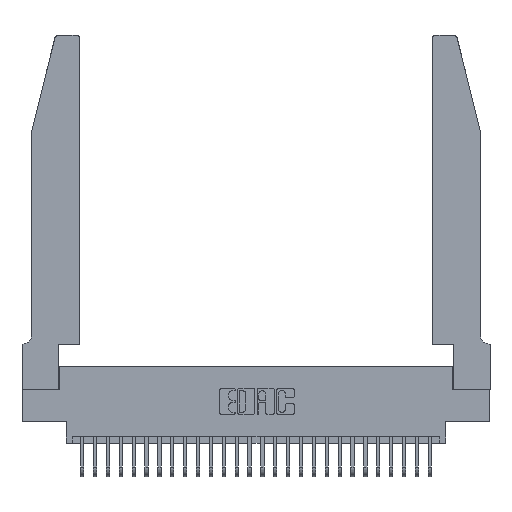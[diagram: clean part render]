
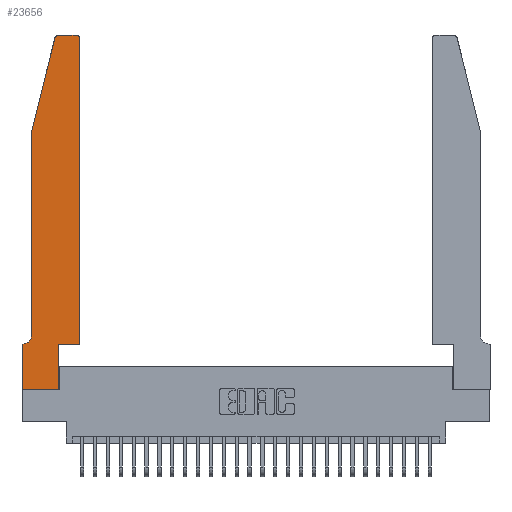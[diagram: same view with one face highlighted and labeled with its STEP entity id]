
A CAD part, top view. The second image highlights one B-rep face of the part: STEP entity #23656.
In plain terms, the highlighted planar face has unit normal (0, 0, 1).
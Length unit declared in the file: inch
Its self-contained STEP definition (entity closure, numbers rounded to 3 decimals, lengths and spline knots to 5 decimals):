
#1052 = DIRECTION ( 'NONE',  ( -1., 0., 0. ) ) ;
#1297 = LINE ( 'NONE', #5480, #9354 ) ;
#1341 = CARTESIAN_POINT ( 'NONE',  ( 0.4505, 0.35, 0.37 ) ) ;
#1685 = EDGE_CURVE ( 'NONE', #15370, #19564, #8620, .T. ) ;
#2724 = CARTESIAN_POINT ( 'NONE',  ( 0.4505, 0.35, 0.37 ) ) ;
#2980 = ORIENTED_EDGE ( 'NONE', *, *, #28537, .T. ) ;
#3102 = CARTESIAN_POINT ( 'NONE',  ( 0.4205, 2.72, 0.37 ) ) ;
#3246 = DIRECTION ( 'NONE',  ( 0., -1., 0. ) ) ;
#3473 = VERTEX_POINT ( 'NONE', #1341 ) ;
#3704 = DIRECTION ( 'NONE',  ( 0., 0., -1. ) ) ;
#3849 = CARTESIAN_POINT ( 'NONE',  ( 0.0755, 2., 0.37 ) ) ;
#4009 = EDGE_CURVE ( 'NONE', #21782, #7893, #15724, .T. ) ;
#4405 = EDGE_CURVE ( 'NONE', #24152, #15370, #26094, .T. ) ;
#5164 = CIRCLE ( 'NONE', #14591, 0.03 ) ;
#5480 = CARTESIAN_POINT ( 'NONE',  ( 0., 0., 0.37 ) ) ;
#5598 = ORIENTED_EDGE ( 'NONE', *, *, #10069, .T. ) ;
#6657 = DIRECTION ( 'NONE',  ( 0., 0., 1. ) ) ;
#6761 = CARTESIAN_POINT ( 'NONE',  ( 0.25487, 2.72718, 0.37 ) ) ;
#6765 = CARTESIAN_POINT ( 'NONE',  ( 0.2865, 0., 0.37 ) ) ;
#7447 = EDGE_CURVE ( 'NONE', #19869, #25562, #26750, .T. ) ;
#7515 = AXIS2_PLACEMENT_3D ( 'NONE', #16096, #20812, #14317 ) ;
#7893 = VERTEX_POINT ( 'NONE', #9432 ) ;
#8620 = LINE ( 'NONE', #20954, #15200 ) ;
#8752 = ORIENTED_EDGE ( 'NONE', *, *, #19323, .T. ) ;
#8914 = AXIS2_PLACEMENT_3D ( 'NONE', #12910, #3704, #1052 ) ;
#8974 = CARTESIAN_POINT ( 'NONE',  ( 0.0755, 0.42, 0.37 ) ) ;
#9147 = CIRCLE ( 'NONE', #8914, 0.07 ) ;
#9189 = CARTESIAN_POINT ( 'NONE',  ( 0.4205, 2.75, 0.37 ) ) ;
#9354 = VECTOR ( 'NONE', #3246, 39.37008 ) ;
#9432 = CARTESIAN_POINT ( 'NONE',  ( 0., 0.35, 0.37 ) ) ;
#9543 = EDGE_CURVE ( 'NONE', #7893, #19869, #1297, .T. ) ;
#9684 = DIRECTION ( 'NONE',  ( 0., 1., 0. ) ) ;
#10012 = VERTEX_POINT ( 'NONE', #9189 ) ;
#10069 = EDGE_CURVE ( 'NONE', #3473, #10582, #26210, .T. ) ;
#10254 = DIRECTION ( 'NONE',  ( 0., 0., 1. ) ) ;
#10582 = VERTEX_POINT ( 'NONE', #24203 ) ;
#11156 = ORIENTED_EDGE ( 'NONE', *, *, #9543, .T. ) ;
#11344 = DIRECTION ( 'NONE',  ( 1., 0., 0. ) ) ;
#11662 = ORIENTED_EDGE ( 'NONE', *, *, #17497, .T. ) ;
#12910 = CARTESIAN_POINT ( 'NONE',  ( 0.0055, 0.42, 0.37 ) ) ;
#14317 = DIRECTION ( 'NONE',  ( 1., 0., 0. ) ) ;
#14591 = AXIS2_PLACEMENT_3D ( 'NONE', #3102, #10254, #21674 ) ;
#14746 = CARTESIAN_POINT ( 'NONE',  ( 0.0755, 2., 0.37 ) ) ;
#14752 = CARTESIAN_POINT ( 'NONE',  ( 0.0755, 0.35, 0.37 ) ) ;
#15053 = DIRECTION ( 'NONE',  ( -1., 0., 0. ) ) ;
#15200 = VECTOR ( 'NONE', #27531, 39.37008 ) ;
#15370 = VERTEX_POINT ( 'NONE', #6761 ) ;
#15724 = LINE ( 'NONE', #14752, #21249 ) ;
#15855 = DIRECTION ( 'NONE',  ( 1., 0., 0. ) ) ;
#16096 = CARTESIAN_POINT ( 'NONE',  ( 0.284, 2.72, 0.37 ) ) ;
#16245 = ORIENTED_EDGE ( 'NONE', *, *, #4405, .T. ) ;
#16783 = VECTOR ( 'NONE', #20620, 39.37008 ) ;
#17304 = LINE ( 'NONE', #30041, #28009 ) ;
#17497 = EDGE_CURVE ( 'NONE', #26085, #21782, #9147, .T. ) ;
#17954 = VECTOR ( 'NONE', #27346, 39.37008 ) ;
#18121 = EDGE_CURVE ( 'NONE', #24529, #3473, #28955, .T. ) ;
#18311 = ORIENTED_EDGE ( 'NONE', *, *, #29194, .T. ) ;
#18580 = CARTESIAN_POINT ( 'NONE',  ( 0.2865, 0.35, 0.37 ) ) ;
#19043 = CARTESIAN_POINT ( 'NONE',  ( 0., 0., 0.37 ) ) ;
#19323 = EDGE_CURVE ( 'NONE', #25562, #24529, #24506, .T. ) ;
#19564 = VERTEX_POINT ( 'NONE', #14746 ) ;
#19869 = VERTEX_POINT ( 'NONE', #22953 ) ;
#19912 = ORIENTED_EDGE ( 'NONE', *, *, #18121, .T. ) ;
#20580 = PLANE ( 'NONE',  #29099 ) ;
#20620 = DIRECTION ( 'NONE',  ( 0., 1., 0. ) ) ;
#20782 = CARTESIAN_POINT ( 'NONE',  ( 0., 0.35, 0.37 ) ) ;
#20812 = DIRECTION ( 'NONE',  ( 0., 0., 1. ) ) ;
#20954 = CARTESIAN_POINT ( 'NONE',  ( 0.0755, 2., 0.37 ) ) ;
#21181 = ORIENTED_EDGE ( 'NONE', *, *, #7447, .T. ) ;
#21249 = VECTOR ( 'NONE', #15053, 39.37008 ) ;
#21520 = DIRECTION ( 'NONE',  ( 1., 0., 0. ) ) ;
#21674 = DIRECTION ( 'NONE',  ( 1., 0., 0. ) ) ;
#21782 = VERTEX_POINT ( 'NONE', #26463 ) ;
#21982 = LINE ( 'NONE', #3849, #17954 ) ;
#22953 = CARTESIAN_POINT ( 'NONE',  ( 0., 0., 0.37 ) ) ;
#22984 = ORIENTED_EDGE ( 'NONE', *, *, #4009, .T. ) ;
#23656 = ADVANCED_FACE ( 'NONE', ( #28815 ), #20580, .T. ) ;
#23783 = VECTOR ( 'NONE', #15855, 39.37008 ) ;
#24152 = VERTEX_POINT ( 'NONE', #25312 ) ;
#24203 = CARTESIAN_POINT ( 'NONE',  ( 0.4505, 2.72, 0.37 ) ) ;
#24231 = CARTESIAN_POINT ( 'NONE',  ( 0.2865, 0.35, 0.37 ) ) ;
#24506 = LINE ( 'NONE', #18580, #16783 ) ;
#24529 = VERTEX_POINT ( 'NONE', #24231 ) ;
#24580 = ORIENTED_EDGE ( 'NONE', *, *, #1685, .T. ) ;
#25312 = CARTESIAN_POINT ( 'NONE',  ( 0.284, 2.75, 0.37 ) ) ;
#25562 = VERTEX_POINT ( 'NONE', #6765 ) ;
#25863 = VECTOR ( 'NONE', #9684, 39.37008 ) ;
#26003 = EDGE_CURVE ( 'NONE', #19564, #26085, #21982, .T. ) ;
#26085 = VERTEX_POINT ( 'NONE', #8974 ) ;
#26094 = CIRCLE ( 'NONE', #7515, 0.03 ) ;
#26210 = LINE ( 'NONE', #2724, #25863 ) ;
#26213 = ORIENTED_EDGE ( 'NONE', *, *, #26003, .T. ) ;
#26463 = CARTESIAN_POINT ( 'NONE',  ( 0.0055, 0.35, 0.37 ) ) ;
#26530 = EDGE_LOOP ( 'NONE', ( #2980, #16245, #24580, #26213, #11662, #22984, #11156, #21181, #8752, #19912, #5598, #18311 ) ) ;
#26538 = DIRECTION ( 'NONE',  ( -1., 0., 0. ) ) ;
#26750 = LINE ( 'NONE', #19043, #28956 ) ;
#27346 = DIRECTION ( 'NONE',  ( 0., -1., 0. ) ) ;
#27531 = DIRECTION ( 'NONE',  ( -0.239, -0.971, 0. ) ) ;
#28009 = VECTOR ( 'NONE', #26538, 39.37008 ) ;
#28537 = EDGE_CURVE ( 'NONE', #10012, #24152, #17304, .T. ) ;
#28815 = FACE_OUTER_BOUND ( 'NONE', #26530, .T. ) ;
#28955 = LINE ( 'NONE', #29941, #23783 ) ;
#28956 = VECTOR ( 'NONE', #21520, 39.37008 ) ;
#29099 = AXIS2_PLACEMENT_3D ( 'NONE', #20782, #6657, #11344 ) ;
#29194 = EDGE_CURVE ( 'NONE', #10582, #10012, #5164, .T. ) ;
#29941 = CARTESIAN_POINT ( 'NONE',  ( 0.4505, 0.35, 0.37 ) ) ;
#30041 = CARTESIAN_POINT ( 'NONE',  ( 0.2605, 2.75, 0.37 ) ) ;
